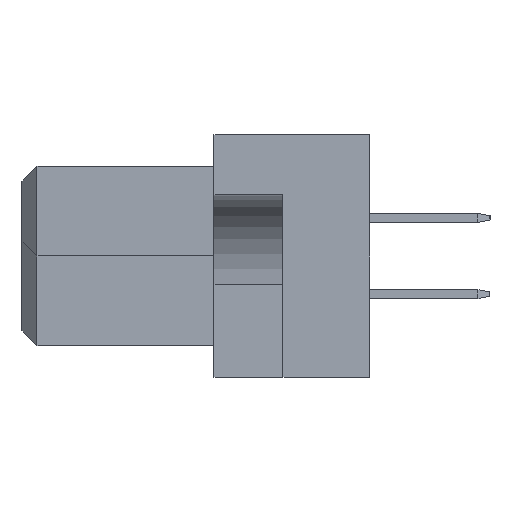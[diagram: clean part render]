
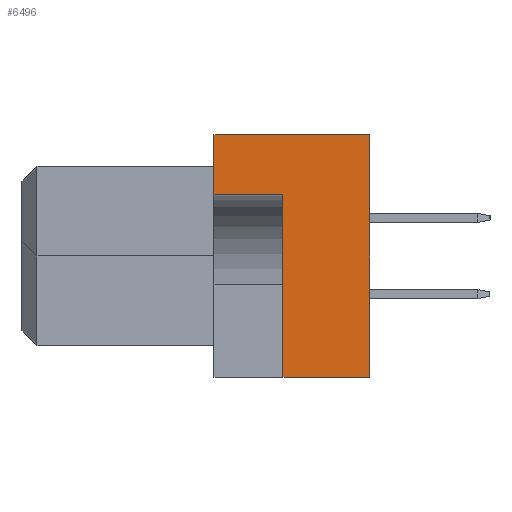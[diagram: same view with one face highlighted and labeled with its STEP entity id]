
A CAD part, left-side view. The second image highlights one B-rep face of the part: STEP entity #6496.
In plain terms, the highlighted planar face has unit normal (-1, 0, 0).
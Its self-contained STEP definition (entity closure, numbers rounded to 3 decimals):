
#89 = CARTESIAN_POINT ( 'NONE',  ( -35.12, 5.2, -4.05 ) ) ;
#536 = CARTESIAN_POINT ( 'NONE',  ( -35.12, 2.9, 2.05 ) ) ;
#1160 = DIRECTION ( 'NONE',  ( 0., 0., 1. ) ) ;
#1180 = DIRECTION ( 'NONE',  ( 0., 0., 1. ) ) ;
#1277 = LINE ( 'NONE', #89, #18318 ) ;
#1346 = ORIENTED_EDGE ( 'NONE', *, *, #3441, .F. ) ;
#1719 = DIRECTION ( 'NONE',  ( 0., 0., 1. ) ) ;
#2596 = ORIENTED_EDGE ( 'NONE', *, *, #13158, .T. ) ;
#3057 = DIRECTION ( 'NONE',  ( 0., 0., -1. ) ) ;
#3098 = CARTESIAN_POINT ( 'NONE',  ( -35.12, 5.2, 4.05 ) ) ;
#3441 = EDGE_CURVE ( 'NONE', #12209, #13826, #7301, .T. ) ;
#4143 = VERTEX_POINT ( 'NONE', #536 ) ;
#4639 = DIRECTION ( 'NONE',  ( 0., -1., 0. ) ) ;
#4652 = VECTOR ( 'NONE', #19194, 1000. ) ;
#5063 = LINE ( 'NONE', #6535, #13294 ) ;
#5155 = VECTOR ( 'NONE', #1180, 1000. ) ;
#6054 = LINE ( 'NONE', #3098, #10551 ) ;
#6496 = ADVANCED_FACE ( 'NONE', ( #10577 ), #7403, .F. ) ;
#6535 = CARTESIAN_POINT ( 'NONE',  ( -35.12, 2.9, 2.05 ) ) ;
#6599 = ORIENTED_EDGE ( 'NONE', *, *, #17005, .F. ) ;
#6852 = DIRECTION ( 'NONE',  ( 0., 1., 0. ) ) ;
#7301 = LINE ( 'NONE', #13141, #4652 ) ;
#7403 = PLANE ( 'NONE',  #16636 ) ;
#7873 = CARTESIAN_POINT ( 'NONE',  ( -35.12, 0., -4.05 ) ) ;
#8032 = ORIENTED_EDGE ( 'NONE', *, *, #9877, .F. ) ;
#8170 = CARTESIAN_POINT ( 'NONE',  ( -35.12, 0., 4.05 ) ) ;
#8254 = EDGE_CURVE ( 'NONE', #12689, #8842, #1277, .T. ) ;
#8671 = VERTEX_POINT ( 'NONE', #17805 ) ;
#8842 = VERTEX_POINT ( 'NONE', #7873 ) ;
#8984 = CARTESIAN_POINT ( 'NONE',  ( -35.12, 5.2, 4.05 ) ) ;
#9105 = CARTESIAN_POINT ( 'NONE',  ( -35.12, 2.9, -4.05 ) ) ;
#9827 = LINE ( 'NONE', #12703, #16822 ) ;
#9877 = EDGE_CURVE ( 'NONE', #12689, #4143, #5063, .T. ) ;
#10551 = VECTOR ( 'NONE', #1719, 1000. ) ;
#10577 = FACE_OUTER_BOUND ( 'NONE', #10591, .T. ) ;
#10591 = EDGE_LOOP ( 'NONE', ( #13486, #6599, #8032, #11037, #2596, #1346 ) ) ;
#11037 = ORIENTED_EDGE ( 'NONE', *, *, #8254, .T. ) ;
#12209 = VERTEX_POINT ( 'NONE', #13309 ) ;
#12689 = VERTEX_POINT ( 'NONE', #9105 ) ;
#12703 = CARTESIAN_POINT ( 'NONE',  ( -35.12, 2.9, 2.05 ) ) ;
#13141 = CARTESIAN_POINT ( 'NONE',  ( -35.12, 5.2, 4.05 ) ) ;
#13158 = EDGE_CURVE ( 'NONE', #8842, #13826, #18125, .T. ) ;
#13255 = DIRECTION ( 'NONE',  ( 1., 0., 0. ) ) ;
#13294 = VECTOR ( 'NONE', #1160, 1000. ) ;
#13309 = CARTESIAN_POINT ( 'NONE',  ( -35.12, 5.2, 4.05 ) ) ;
#13486 = ORIENTED_EDGE ( 'NONE', *, *, #18575, .F. ) ;
#13826 = VERTEX_POINT ( 'NONE', #8170 ) ;
#16636 = AXIS2_PLACEMENT_3D ( 'NONE', #8984, #13255, #3057 ) ;
#16822 = VECTOR ( 'NONE', #6852, 1000. ) ;
#17005 = EDGE_CURVE ( 'NONE', #4143, #8671, #9827, .T. ) ;
#17805 = CARTESIAN_POINT ( 'NONE',  ( -35.12, 5.2, 2.05 ) ) ;
#18125 = LINE ( 'NONE', #19411, #5155 ) ;
#18318 = VECTOR ( 'NONE', #4639, 1000. ) ;
#18575 = EDGE_CURVE ( 'NONE', #8671, #12209, #6054, .T. ) ;
#19194 = DIRECTION ( 'NONE',  ( 0., -1., 0. ) ) ;
#19411 = CARTESIAN_POINT ( 'NONE',  ( -35.12, 0., 4.05 ) ) ;
